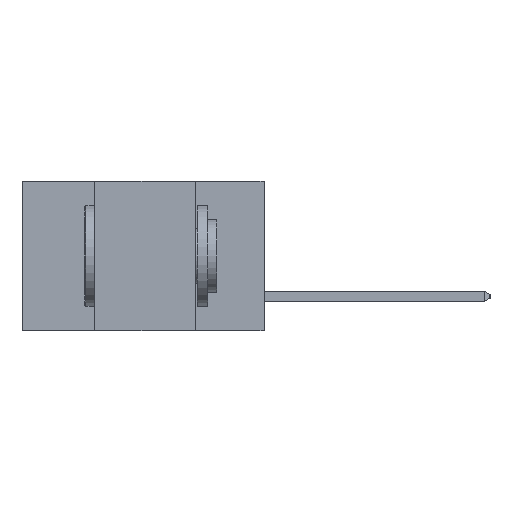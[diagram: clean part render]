
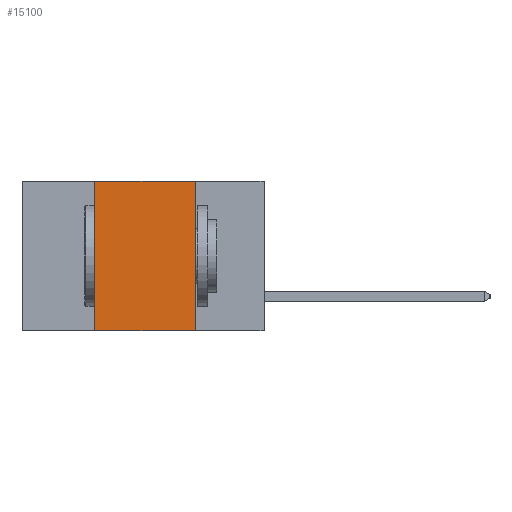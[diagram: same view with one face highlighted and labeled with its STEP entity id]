
A CAD part, left-side view. The second image highlights one B-rep face of the part: STEP entity #15100.
In plain terms, the highlighted planar face has unit normal (-1, 0, 0).
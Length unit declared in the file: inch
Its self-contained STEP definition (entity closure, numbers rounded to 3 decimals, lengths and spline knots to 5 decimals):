
#341 = CARTESIAN_POINT ( 'NONE',  ( 0., 0.6, 0. ) ) ;
#726 = EDGE_CURVE ( 'NONE', #3400, #2053, #8045, .T. ) ;
#980 = CARTESIAN_POINT ( 'NONE',  ( 0., 0.42, -0.37 ) ) ;
#1160 = VERTEX_POINT ( 'NONE', #5290 ) ;
#2053 = VERTEX_POINT ( 'NONE', #6286 ) ;
#2133 = ORIENTED_EDGE ( 'NONE', *, *, #4159, .F. ) ;
#2921 = DIRECTION ( 'NONE',  ( 0., 0., -1. ) ) ;
#3306 = EDGE_CURVE ( 'NONE', #3400, #1160, #12285, .T. ) ;
#3400 = VERTEX_POINT ( 'NONE', #980 ) ;
#3525 = AXIS2_PLACEMENT_3D ( 'NONE', #341, #10016, #2921 ) ;
#3706 = DIRECTION ( 'NONE',  ( 0., 0., 1. ) ) ;
#4159 = EDGE_CURVE ( 'NONE', #1160, #4987, #13340, .T. ) ;
#4234 = CARTESIAN_POINT ( 'NONE',  ( 0., 0.42, -0.37 ) ) ;
#4685 = ORIENTED_EDGE ( 'NONE', *, *, #726, .T. ) ;
#4982 = EDGE_CURVE ( 'NONE', #4987, #2053, #5151, .T. ) ;
#4987 = VERTEX_POINT ( 'NONE', #13316 ) ;
#5151 = LINE ( 'NONE', #5155, #10955 ) ;
#5155 = CARTESIAN_POINT ( 'NONE',  ( 0., 0.17, -0.37 ) ) ;
#5257 = FACE_OUTER_BOUND ( 'NONE', #8340, .T. ) ;
#5290 = CARTESIAN_POINT ( 'NONE',  ( 0., 0.42, 0. ) ) ;
#6109 = VECTOR ( 'NONE', #3706, 39.37008 ) ;
#6286 = CARTESIAN_POINT ( 'NONE',  ( 0., 0.17, -0.37 ) ) ;
#6778 = ORIENTED_EDGE ( 'NONE', *, *, #3306, .F. ) ;
#7143 = VECTOR ( 'NONE', #14457, 39.37008 ) ;
#7674 = PLANE ( 'NONE',  #3525 ) ;
#7975 = ORIENTED_EDGE ( 'NONE', *, *, #4982, .F. ) ;
#8045 = LINE ( 'NONE', #9536, #13525 ) ;
#8340 = EDGE_LOOP ( 'NONE', ( #7975, #2133, #6778, #4685 ) ) ;
#9490 = DIRECTION ( 'NONE',  ( 0., -1., 0. ) ) ;
#9536 = CARTESIAN_POINT ( 'NONE',  ( 0., 0.6, -0.37 ) ) ;
#10016 = DIRECTION ( 'NONE',  ( 1., 0., 0. ) ) ;
#10955 = VECTOR ( 'NONE', #12151, 39.37008 ) ;
#12151 = DIRECTION ( 'NONE',  ( 0., 0., -1. ) ) ;
#12285 = LINE ( 'NONE', #4234, #6109 ) ;
#13316 = CARTESIAN_POINT ( 'NONE',  ( 0., 0.17, 0. ) ) ;
#13340 = LINE ( 'NONE', #14744, #7143 ) ;
#13525 = VECTOR ( 'NONE', #9490, 39.37008 ) ;
#14457 = DIRECTION ( 'NONE',  ( 0., -1., 0. ) ) ;
#14744 = CARTESIAN_POINT ( 'NONE',  ( 0., 0.6, 0. ) ) ;
#15100 = ADVANCED_FACE ( 'NONE', ( #5257 ), #7674, .F. ) ;
